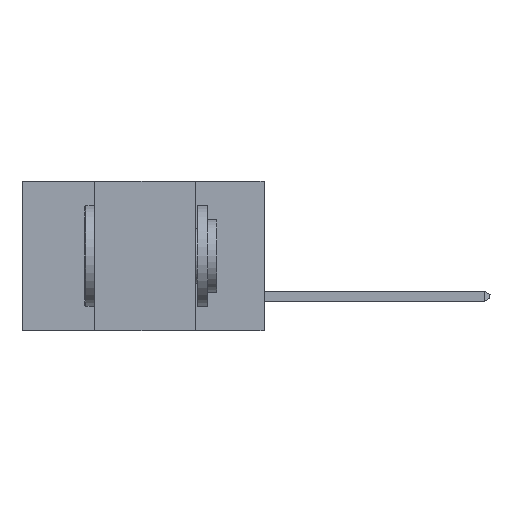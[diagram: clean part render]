
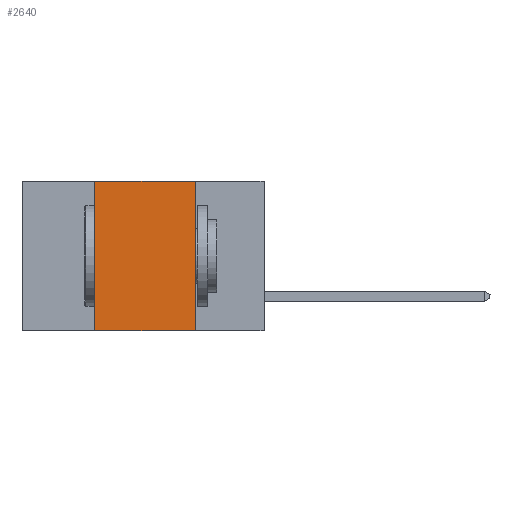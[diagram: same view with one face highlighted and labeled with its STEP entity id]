
A CAD part, left-side view. The second image highlights one B-rep face of the part: STEP entity #2640.
In plain terms, the highlighted planar face has unit normal (-1, 0, 0).
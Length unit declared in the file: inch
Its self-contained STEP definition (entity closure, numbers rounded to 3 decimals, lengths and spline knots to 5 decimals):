
#741 = CARTESIAN_POINT ( 'NONE',  ( 0., 0.42, -0.37 ) ) ;
#931 = CARTESIAN_POINT ( 'NONE',  ( 0., 0.6, 0. ) ) ;
#1035 = VECTOR ( 'NONE', #1250, 39.37008 ) ;
#1250 = DIRECTION ( 'NONE',  ( 0., 0., 1. ) ) ;
#1323 = CARTESIAN_POINT ( 'NONE',  ( 0., 0.42, 0. ) ) ;
#1554 = CARTESIAN_POINT ( 'NONE',  ( 0., 0.17, 0. ) ) ;
#2139 = LINE ( 'NONE', #1323, #1035 ) ;
#2640 = ADVANCED_FACE ( 'NONE', ( #13453 ), #8525, .F. ) ;
#3238 = LINE ( 'NONE', #5173, #21405 ) ;
#5039 = ORIENTED_EDGE ( 'NONE', *, *, #9897, .T. ) ;
#5173 = CARTESIAN_POINT ( 'NONE',  ( 0., 0.17, 0. ) ) ;
#5222 = DIRECTION ( 'NONE',  ( 1., 0., 0. ) ) ;
#5301 = VERTEX_POINT ( 'NONE', #741 ) ;
#5898 = ORIENTED_EDGE ( 'NONE', *, *, #8252, .F. ) ;
#6958 = VECTOR ( 'NONE', #20357, 39.37008 ) ;
#8158 = VERTEX_POINT ( 'NONE', #1554 ) ;
#8251 = ORIENTED_EDGE ( 'NONE', *, *, #21848, .F. ) ;
#8252 = EDGE_CURVE ( 'NONE', #5301, #8721, #2139, .T. ) ;
#8312 = AXIS2_PLACEMENT_3D ( 'NONE', #8747, #5222, #21137 ) ;
#8525 = PLANE ( 'NONE',  #8312 ) ;
#8549 = DIRECTION ( 'NONE',  ( 0., 0., -1. ) ) ;
#8622 = ORIENTED_EDGE ( 'NONE', *, *, #11082, .F. ) ;
#8721 = VERTEX_POINT ( 'NONE', #22031 ) ;
#8747 = CARTESIAN_POINT ( 'NONE',  ( 0., 0.6, 0. ) ) ;
#8836 = CARTESIAN_POINT ( 'NONE',  ( 0., 0.17, -0.37 ) ) ;
#9897 = EDGE_CURVE ( 'NONE', #5301, #18301, #17432, .T. ) ;
#11078 = EDGE_LOOP ( 'NONE', ( #8251, #8622, #5898, #5039 ) ) ;
#11082 = EDGE_CURVE ( 'NONE', #8721, #8158, #22360, .T. ) ;
#13453 = FACE_OUTER_BOUND ( 'NONE', #11078, .T. ) ;
#15012 = CARTESIAN_POINT ( 'NONE',  ( 0., 0.6, -0.37 ) ) ;
#16752 = DIRECTION ( 'NONE',  ( 0., -1., 0. ) ) ;
#16866 = VECTOR ( 'NONE', #16752, 39.37008 ) ;
#17432 = LINE ( 'NONE', #15012, #16866 ) ;
#18301 = VERTEX_POINT ( 'NONE', #8836 ) ;
#20357 = DIRECTION ( 'NONE',  ( 0., -1., 0. ) ) ;
#21137 = DIRECTION ( 'NONE',  ( 0., 0., -1. ) ) ;
#21405 = VECTOR ( 'NONE', #8549, 39.37008 ) ;
#21848 = EDGE_CURVE ( 'NONE', #8158, #18301, #3238, .T. ) ;
#22031 = CARTESIAN_POINT ( 'NONE',  ( 0., 0.42, 0. ) ) ;
#22360 = LINE ( 'NONE', #931, #6958 ) ;
